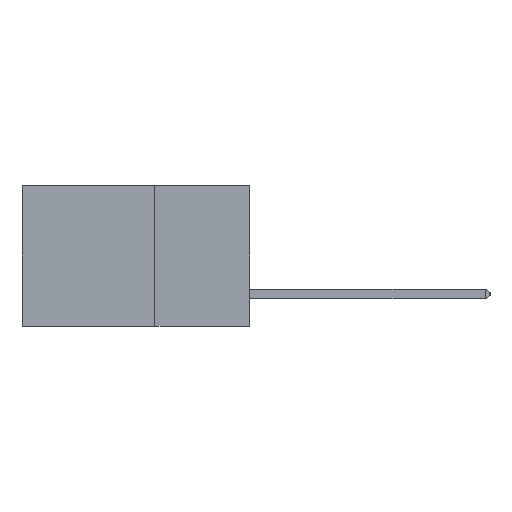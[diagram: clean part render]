
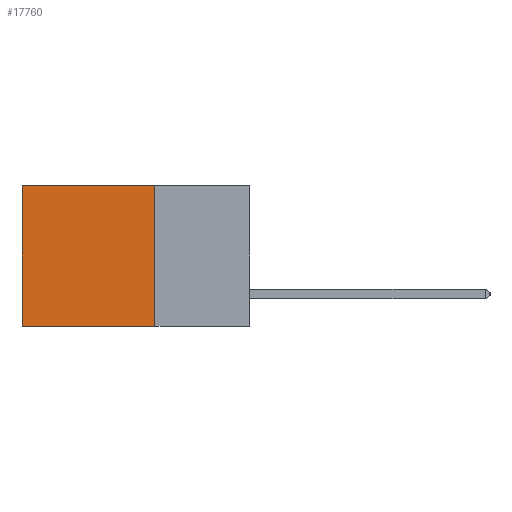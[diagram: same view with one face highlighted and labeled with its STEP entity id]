
A CAD part, left-side view. The second image highlights one B-rep face of the part: STEP entity #17760.
In plain terms, the highlighted planar face has unit normal (-1, 0, 0).
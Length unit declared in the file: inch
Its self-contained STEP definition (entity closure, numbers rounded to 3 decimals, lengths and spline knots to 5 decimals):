
#237 = CARTESIAN_POINT ( 'NONE',  ( 0.2875, 0.6, -0.37 ) ) ;
#727 = DIRECTION ( 'NONE',  ( 1., 0., 0. ) ) ;
#972 = CARTESIAN_POINT ( 'NONE',  ( 0.2875, 0.25, -0.37 ) ) ;
#1492 = VECTOR ( 'NONE', #8671, 39.37008 ) ;
#2252 = ORIENTED_EDGE ( 'NONE', *, *, #22095, .T. ) ;
#2285 = VECTOR ( 'NONE', #16361, 39.37008 ) ;
#2306 = EDGE_LOOP ( 'NONE', ( #9223, #14003, #8776, #2252 ) ) ;
#3505 = LINE ( 'NONE', #18093, #8295 ) ;
#4468 = CARTESIAN_POINT ( 'NONE',  ( 0.2875, 0.25, 0. ) ) ;
#5304 = CARTESIAN_POINT ( 'NONE',  ( 0.2875, 0.6, 0. ) ) ;
#6963 = LINE ( 'NONE', #4468, #1492 ) ;
#8295 = VECTOR ( 'NONE', #14136, 39.37008 ) ;
#8671 = DIRECTION ( 'NONE',  ( 0., 0., -1. ) ) ;
#8776 = ORIENTED_EDGE ( 'NONE', *, *, #18984, .F. ) ;
#8919 = CARTESIAN_POINT ( 'NONE',  ( 0.2875, 0.25, 0. ) ) ;
#9223 = ORIENTED_EDGE ( 'NONE', *, *, #13168, .T. ) ;
#10279 = VERTEX_POINT ( 'NONE', #237 ) ;
#12070 = CARTESIAN_POINT ( 'NONE',  ( 0.2875, 0.25, 0. ) ) ;
#13168 = EDGE_CURVE ( 'NONE', #16910, #10279, #25397, .T. ) ;
#13267 = LINE ( 'NONE', #12070, #2285 ) ;
#13941 = CARTESIAN_POINT ( 'NONE',  ( 0.2875, 0.25, 0. ) ) ;
#14003 = ORIENTED_EDGE ( 'NONE', *, *, #16340, .F. ) ;
#14136 = DIRECTION ( 'NONE',  ( 0., 1., 0. ) ) ;
#15191 = DIRECTION ( 'NONE',  ( 0., 0., -1. ) ) ;
#16280 = VERTEX_POINT ( 'NONE', #13941 ) ;
#16340 = EDGE_CURVE ( 'NONE', #18478, #10279, #3505, .T. ) ;
#16361 = DIRECTION ( 'NONE',  ( 0., 1., 0. ) ) ;
#16910 = VERTEX_POINT ( 'NONE', #24519 ) ;
#17161 = PLANE ( 'NONE',  #25562 ) ;
#17760 = ADVANCED_FACE ( 'NONE', ( #26271 ), #17161, .F. ) ;
#18093 = CARTESIAN_POINT ( 'NONE',  ( 0.2875, 0.25, -0.37 ) ) ;
#18478 = VERTEX_POINT ( 'NONE', #972 ) ;
#18984 = EDGE_CURVE ( 'NONE', #16280, #18478, #6963, .T. ) ;
#21867 = DIRECTION ( 'NONE',  ( 0., 0., -1. ) ) ;
#22095 = EDGE_CURVE ( 'NONE', #16280, #16910, #13267, .T. ) ;
#24122 = VECTOR ( 'NONE', #21867, 39.37008 ) ;
#24519 = CARTESIAN_POINT ( 'NONE',  ( 0.2875, 0.6, 0. ) ) ;
#25397 = LINE ( 'NONE', #5304, #24122 ) ;
#25562 = AXIS2_PLACEMENT_3D ( 'NONE', #8919, #727, #15191 ) ;
#26271 = FACE_OUTER_BOUND ( 'NONE', #2306, .T. ) ;
